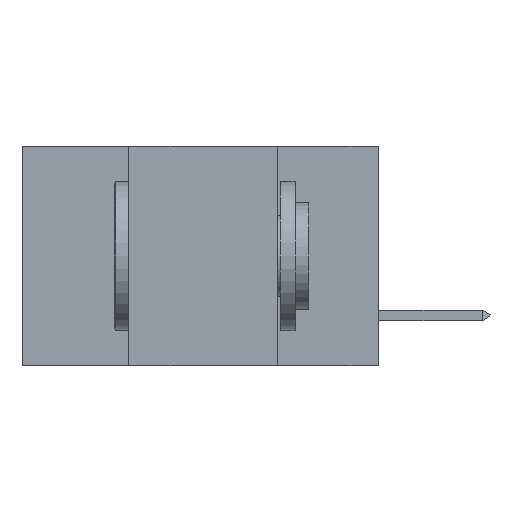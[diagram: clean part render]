
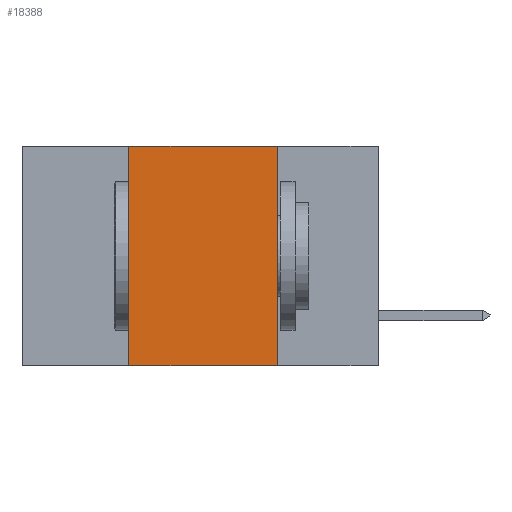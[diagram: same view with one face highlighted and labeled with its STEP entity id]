
A CAD part, left-side view. The second image highlights one B-rep face of the part: STEP entity #18388.
In plain terms, the highlighted planar face has unit normal (-1, 0, 0).
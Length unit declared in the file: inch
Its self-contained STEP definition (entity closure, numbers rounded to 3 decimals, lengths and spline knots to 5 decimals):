
#328 = DIRECTION ( 'NONE',  ( 0., -1., 0. ) ) ;
#451 = CARTESIAN_POINT ( 'NONE',  ( 0., 0.6, 0. ) ) ;
#1200 = DIRECTION ( 'NONE',  ( 0., 0., 1. ) ) ;
#1302 = CARTESIAN_POINT ( 'NONE',  ( 0., 0.42, 0. ) ) ;
#2042 = VECTOR ( 'NONE', #328, 39.37008 ) ;
#4579 = VERTEX_POINT ( 'NONE', #24870 ) ;
#4820 = EDGE_CURVE ( 'NONE', #29967, #17393, #9388, .T. ) ;
#6378 = EDGE_LOOP ( 'NONE', ( #21320, #15236, #28972, #22659 ) ) ;
#7050 = CARTESIAN_POINT ( 'NONE',  ( 0., 0.17, 0. ) ) ;
#8427 = EDGE_CURVE ( 'NONE', #8975, #29967, #13622, .T. ) ;
#8975 = VERTEX_POINT ( 'NONE', #28714 ) ;
#9388 = LINE ( 'NONE', #7050, #26886 ) ;
#10266 = CARTESIAN_POINT ( 'NONE',  ( 0., 0.17, 0. ) ) ;
#10463 = EDGE_CURVE ( 'NONE', #4579, #17393, #24560, .T. ) ;
#12324 = DIRECTION ( 'NONE',  ( 1., 0., 0. ) ) ;
#13622 = LINE ( 'NONE', #19584, #2042 ) ;
#14092 = FACE_OUTER_BOUND ( 'NONE', #6378, .T. ) ;
#14455 = VECTOR ( 'NONE', #21509, 39.37008 ) ;
#15236 = ORIENTED_EDGE ( 'NONE', *, *, #8427, .F. ) ;
#17011 = DIRECTION ( 'NONE',  ( 0., 0., -1. ) ) ;
#17393 = VERTEX_POINT ( 'NONE', #22716 ) ;
#18388 = ADVANCED_FACE ( 'NONE', ( #14092 ), #26405, .F. ) ;
#19584 = CARTESIAN_POINT ( 'NONE',  ( 0., 0.6, 0. ) ) ;
#19693 = AXIS2_PLACEMENT_3D ( 'NONE', #451, #12324, #17011 ) ;
#21320 = ORIENTED_EDGE ( 'NONE', *, *, #4820, .F. ) ;
#21509 = DIRECTION ( 'NONE',  ( 0., -1., 0. ) ) ;
#22659 = ORIENTED_EDGE ( 'NONE', *, *, #10463, .T. ) ;
#22716 = CARTESIAN_POINT ( 'NONE',  ( 0., 0.17, -0.37 ) ) ;
#23219 = VECTOR ( 'NONE', #1200, 39.37008 ) ;
#24560 = LINE ( 'NONE', #30410, #14455 ) ;
#24702 = LINE ( 'NONE', #1302, #23219 ) ;
#24870 = CARTESIAN_POINT ( 'NONE',  ( 0., 0.42, -0.37 ) ) ;
#25858 = EDGE_CURVE ( 'NONE', #4579, #8975, #24702, .T. ) ;
#26405 = PLANE ( 'NONE',  #19693 ) ;
#26886 = VECTOR ( 'NONE', #28816, 39.37008 ) ;
#28714 = CARTESIAN_POINT ( 'NONE',  ( 0., 0.42, 0. ) ) ;
#28816 = DIRECTION ( 'NONE',  ( 0., 0., -1. ) ) ;
#28972 = ORIENTED_EDGE ( 'NONE', *, *, #25858, .F. ) ;
#29967 = VERTEX_POINT ( 'NONE', #10266 ) ;
#30410 = CARTESIAN_POINT ( 'NONE',  ( 0., 0.6, -0.37 ) ) ;
